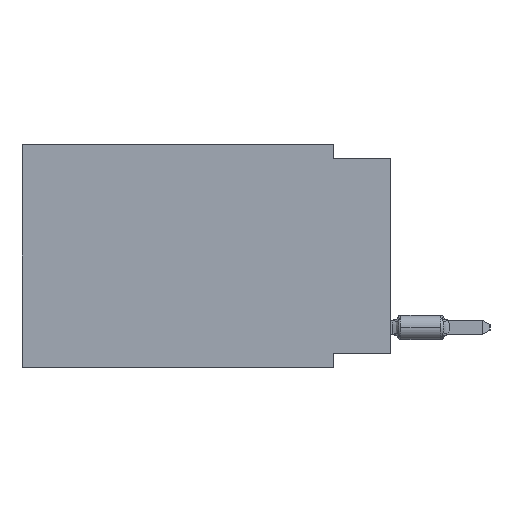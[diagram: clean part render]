
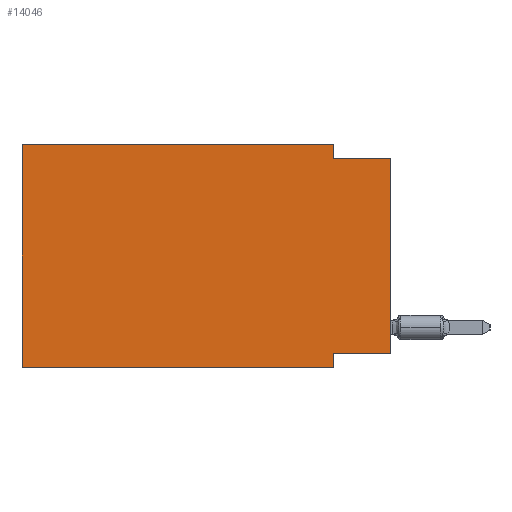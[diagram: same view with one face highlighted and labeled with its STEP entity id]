
A CAD part, left-side view. The second image highlights one B-rep face of the part: STEP entity #14046.
In plain terms, the highlighted planar face has unit normal (-1, 0, 0).
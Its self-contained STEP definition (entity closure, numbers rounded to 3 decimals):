
#314 = VERTEX_POINT ( 'NONE', #15193 ) ;
#455 = VERTEX_POINT ( 'NONE', #17210 ) ;
#653 = VECTOR ( 'NONE', #17330, 1000. ) ;
#856 = VERTEX_POINT ( 'NONE', #20307 ) ;
#1063 = CARTESIAN_POINT ( 'NONE',  ( 0., 16.383, 0. ) ) ;
#1074 = VERTEX_POINT ( 'NONE', #21416 ) ;
#1121 = VECTOR ( 'NONE', #8066, 1000. ) ;
#1277 = EDGE_CURVE ( 'NONE', #7307, #12651, #4794, .T. ) ;
#1327 = DIRECTION ( 'NONE',  ( 1., 0., 0. ) ) ;
#1657 = DIRECTION ( 'NONE',  ( 0., 0., -1. ) ) ;
#2418 = DIRECTION ( 'NONE',  ( 0., -1., 0. ) ) ;
#3576 = LINE ( 'NONE', #15762, #7993 ) ;
#3660 = EDGE_CURVE ( 'NONE', #12651, #856, #17347, .T. ) ;
#4019 = AXIS2_PLACEMENT_3D ( 'NONE', #4943, #1327, #1657 ) ;
#4456 = CARTESIAN_POINT ( 'NONE',  ( 0., 16.383, -9.906 ) ) ;
#4794 = LINE ( 'NONE', #15073, #1121 ) ;
#4823 = VECTOR ( 'NONE', #22262, 1000. ) ;
#4943 = CARTESIAN_POINT ( 'NONE',  ( 0., 16.383, 0. ) ) ;
#5734 = LINE ( 'NONE', #10828, #16787 ) ;
#6060 = ORIENTED_EDGE ( 'NONE', *, *, #15949, .T. ) ;
#6065 = ORIENTED_EDGE ( 'NONE', *, *, #1277, .F. ) ;
#6279 = EDGE_CURVE ( 'NONE', #1074, #7307, #8629, .T. ) ;
#6897 = VECTOR ( 'NONE', #2418, 1000. ) ;
#7234 = CARTESIAN_POINT ( 'NONE',  ( 0., 2.54, -0.635 ) ) ;
#7303 = ORIENTED_EDGE ( 'NONE', *, *, #13377, .F. ) ;
#7307 = VERTEX_POINT ( 'NONE', #12560 ) ;
#7506 = VECTOR ( 'NONE', #13736, 1000. ) ;
#7612 = ORIENTED_EDGE ( 'NONE', *, *, #6279, .F. ) ;
#7993 = VECTOR ( 'NONE', #20545, 1000. ) ;
#8066 = DIRECTION ( 'NONE',  ( 0., 0., -1. ) ) ;
#8076 = ORIENTED_EDGE ( 'NONE', *, *, #11908, .T. ) ;
#8081 = LINE ( 'NONE', #1063, #17789 ) ;
#8495 = ORIENTED_EDGE ( 'NONE', *, *, #3660, .F. ) ;
#8629 = LINE ( 'NONE', #9058, #653 ) ;
#9058 = CARTESIAN_POINT ( 'NONE',  ( 0., 16.383, 0. ) ) ;
#10231 = CARTESIAN_POINT ( 'NONE',  ( 0., 0., -0.635 ) ) ;
#10828 = CARTESIAN_POINT ( 'NONE',  ( 0., 2.54, -9.906 ) ) ;
#11738 = CARTESIAN_POINT ( 'NONE',  ( 0., 0., -9.271 ) ) ;
#11908 = EDGE_CURVE ( 'NONE', #18461, #856, #3576, .T. ) ;
#12560 = CARTESIAN_POINT ( 'NONE',  ( 0., 2.54, 0. ) ) ;
#12651 = VERTEX_POINT ( 'NONE', #7234 ) ;
#13377 = EDGE_CURVE ( 'NONE', #18461, #314, #15349, .T. ) ;
#13736 = DIRECTION ( 'NONE',  ( 0., -1., 0. ) ) ;
#14046 = ADVANCED_FACE ( 'NONE', ( #17036 ), #17143, .F. ) ;
#14131 = ORIENTED_EDGE ( 'NONE', *, *, #16378, .F. ) ;
#15073 = CARTESIAN_POINT ( 'NONE',  ( 0., 2.54, 0. ) ) ;
#15193 = CARTESIAN_POINT ( 'NONE',  ( 0., 2.54, -9.271 ) ) ;
#15349 = LINE ( 'NONE', #11738, #4823 ) ;
#15762 = CARTESIAN_POINT ( 'NONE',  ( 0., 0., 0. ) ) ;
#15949 = EDGE_CURVE ( 'NONE', #21656, #455, #19304, .T. ) ;
#16378 = EDGE_CURVE ( 'NONE', #314, #455, #5734, .T. ) ;
#16787 = VECTOR ( 'NONE', #17729, 1000. ) ;
#17036 = FACE_OUTER_BOUND ( 'NONE', #19642, .T. ) ;
#17143 = PLANE ( 'NONE',  #4019 ) ;
#17210 = CARTESIAN_POINT ( 'NONE',  ( 0., 2.54, -9.906 ) ) ;
#17330 = DIRECTION ( 'NONE',  ( 0., -1., 0. ) ) ;
#17347 = LINE ( 'NONE', #10231, #7506 ) ;
#17597 = CARTESIAN_POINT ( 'NONE',  ( 0., 16.383, -9.906 ) ) ;
#17729 = DIRECTION ( 'NONE',  ( 0., 0., -1. ) ) ;
#17789 = VECTOR ( 'NONE', #18591, 1000. ) ;
#18255 = ORIENTED_EDGE ( 'NONE', *, *, #21599, .F. ) ;
#18461 = VERTEX_POINT ( 'NONE', #18753 ) ;
#18591 = DIRECTION ( 'NONE',  ( 0., 0., 1. ) ) ;
#18753 = CARTESIAN_POINT ( 'NONE',  ( 0., 0., -9.271 ) ) ;
#19304 = LINE ( 'NONE', #17597, #6897 ) ;
#19642 = EDGE_LOOP ( 'NONE', ( #8076, #8495, #6065, #7612, #18255, #6060, #14131, #7303 ) ) ;
#20307 = CARTESIAN_POINT ( 'NONE',  ( 0., 0., -0.635 ) ) ;
#20545 = DIRECTION ( 'NONE',  ( 0., 0., 1. ) ) ;
#21416 = CARTESIAN_POINT ( 'NONE',  ( 0., 16.383, 0. ) ) ;
#21599 = EDGE_CURVE ( 'NONE', #21656, #1074, #8081, .T. ) ;
#21656 = VERTEX_POINT ( 'NONE', #4456 ) ;
#22262 = DIRECTION ( 'NONE',  ( 0., 1., 0. ) ) ;
